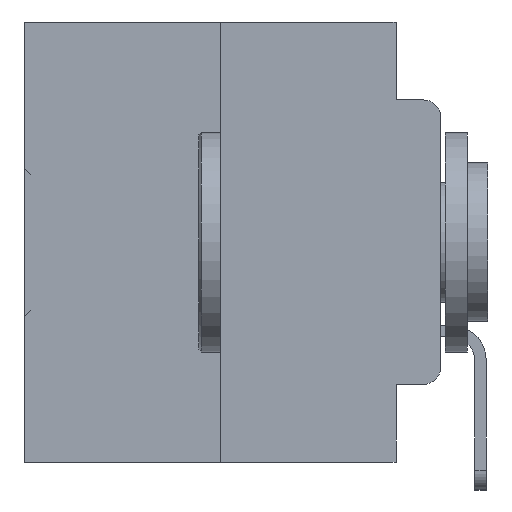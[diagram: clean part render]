
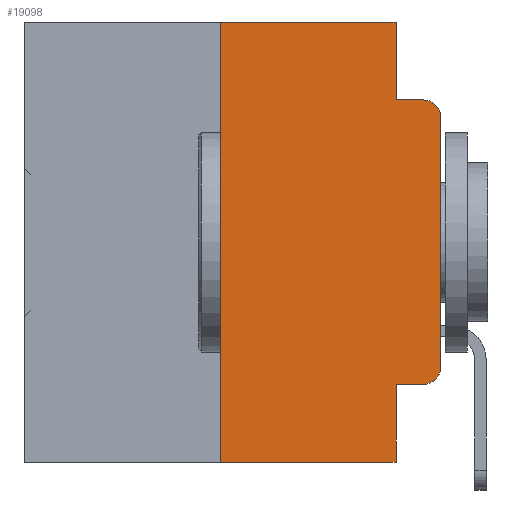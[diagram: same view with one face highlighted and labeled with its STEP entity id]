
A CAD part, left-side view. The second image highlights one B-rep face of the part: STEP entity #19098.
In plain terms, the highlighted planar face has unit normal (-1, 0, 0).
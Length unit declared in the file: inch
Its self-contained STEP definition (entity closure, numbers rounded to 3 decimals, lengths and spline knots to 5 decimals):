
#372 = AXIS2_PLACEMENT_3D ( 'NONE', #493, #19734, #3300 ) ;
#493 = CARTESIAN_POINT ( 'NONE',  ( 0., 0.02, -0.1085 ) ) ;
#809 = DIRECTION ( 'NONE',  ( 0., -1., 0. ) ) ;
#1247 = CARTESIAN_POINT ( 'NONE',  ( 0., 0.25, 0. ) ) ;
#1377 = DIRECTION ( 'NONE',  ( 0., 0., -1. ) ) ;
#1588 = DIRECTION ( 'NONE',  ( 0., 0., -1. ) ) ;
#1633 = CARTESIAN_POINT ( 'NONE',  ( 0., 0.051, -0.0885 ) ) ;
#1712 = CARTESIAN_POINT ( 'NONE',  ( 0., 0.051, 0. ) ) ;
#2643 = AXIS2_PLACEMENT_3D ( 'NONE', #33662, #17865, #1377 ) ;
#2871 = VERTEX_POINT ( 'NONE', #22333 ) ;
#2929 = DIRECTION ( 'NONE',  ( 0., 0., -1. ) ) ;
#3300 = DIRECTION ( 'NONE',  ( 0., 0., -1. ) ) ;
#3422 = EDGE_LOOP ( 'NONE', ( #8498, #23719, #23021, #17663, #18103, #30913, #30508, #13424, #20625, #8719 ) ) ;
#4654 = CARTESIAN_POINT ( 'NONE',  ( 0., 0.02, -0.4115 ) ) ;
#4959 = CARTESIAN_POINT ( 'NONE',  ( 0., 0.051, -0.5 ) ) ;
#5313 = DIRECTION ( 'NONE',  ( 0., -1., 0. ) ) ;
#5554 = DIRECTION ( 'NONE',  ( 0., 0., -1. ) ) ;
#5927 = VERTEX_POINT ( 'NONE', #18514 ) ;
#6428 = CARTESIAN_POINT ( 'NONE',  ( 0., 0.473, -0.5 ) ) ;
#8099 = CARTESIAN_POINT ( 'NONE',  ( 0., 0.473, 0. ) ) ;
#8263 = CARTESIAN_POINT ( 'NONE',  ( 0., 0.473, 0. ) ) ;
#8498 = ORIENTED_EDGE ( 'NONE', *, *, #14385, .T. ) ;
#8561 = VERTEX_POINT ( 'NONE', #28692 ) ;
#8691 = VERTEX_POINT ( 'NONE', #4959 ) ;
#8719 = ORIENTED_EDGE ( 'NONE', *, *, #18761, .T. ) ;
#9183 = VERTEX_POINT ( 'NONE', #18620 ) ;
#10094 = VERTEX_POINT ( 'NONE', #1633 ) ;
#10362 = LINE ( 'NONE', #30928, #16781 ) ;
#10534 = VECTOR ( 'NONE', #1588, 39.37008 ) ;
#10754 = EDGE_CURVE ( 'NONE', #10094, #27818, #10362, .T. ) ;
#11478 = LINE ( 'NONE', #16391, #26593 ) ;
#11793 = LINE ( 'NONE', #14503, #32259 ) ;
#12131 = CARTESIAN_POINT ( 'NONE',  ( 0., 0.25, 0. ) ) ;
#12580 = EDGE_CURVE ( 'NONE', #5927, #27818, #28372, .T. ) ;
#13424 = ORIENTED_EDGE ( 'NONE', *, *, #27581, .F. ) ;
#14385 = EDGE_CURVE ( 'NONE', #8561, #5927, #11478, .T. ) ;
#14503 = CARTESIAN_POINT ( 'NONE',  ( 0., 0.051, -0.4115 ) ) ;
#14835 = AXIS2_PLACEMENT_3D ( 'NONE', #8263, #19368, #2929 ) ;
#15530 = EDGE_CURVE ( 'NONE', #23716, #8691, #27016, .T. ) ;
#16251 = CIRCLE ( 'NONE', #2643, 0.02 ) ;
#16391 = CARTESIAN_POINT ( 'NONE',  ( 0., 0., 0. ) ) ;
#16655 = PLANE ( 'NONE',  #14835 ) ;
#16781 = VECTOR ( 'NONE', #17764, 39.37008 ) ;
#16973 = VECTOR ( 'NONE', #5554, 39.37008 ) ;
#17362 = VECTOR ( 'NONE', #5313, 39.37008 ) ;
#17663 = ORIENTED_EDGE ( 'NONE', *, *, #34643, .F. ) ;
#17764 = DIRECTION ( 'NONE',  ( 0., -1., 0. ) ) ;
#17814 = LINE ( 'NONE', #1712, #10534 ) ;
#17865 = DIRECTION ( 'NONE',  ( -1., 0., 0. ) ) ;
#18103 = ORIENTED_EDGE ( 'NONE', *, *, #34859, .F. ) ;
#18493 = LINE ( 'NONE', #1247, #30865 ) ;
#18514 = CARTESIAN_POINT ( 'NONE',  ( 0., 0., -0.1085 ) ) ;
#18620 = CARTESIAN_POINT ( 'NONE',  ( 0., 0.051, -0.4115 ) ) ;
#18761 = EDGE_CURVE ( 'NONE', #20790, #8561, #16251, .T. ) ;
#19098 = ADVANCED_FACE ( 'NONE', ( #24135 ), #16655, .F. ) ;
#19368 = DIRECTION ( 'NONE',  ( 1., 0., 0. ) ) ;
#19734 = DIRECTION ( 'NONE',  ( -1., 0., 0. ) ) ;
#19964 = DIRECTION ( 'NONE',  ( 0., -1., 0. ) ) ;
#20534 = EDGE_CURVE ( 'NONE', #9183, #20790, #11793, .T. ) ;
#20625 = ORIENTED_EDGE ( 'NONE', *, *, #20534, .T. ) ;
#20790 = VERTEX_POINT ( 'NONE', #4654 ) ;
#22333 = CARTESIAN_POINT ( 'NONE',  ( 0., 0.051, 0. ) ) ;
#23021 = ORIENTED_EDGE ( 'NONE', *, *, #10754, .F. ) ;
#23048 = CARTESIAN_POINT ( 'NONE',  ( 0., 0.25, -0.5 ) ) ;
#23716 = VERTEX_POINT ( 'NONE', #23048 ) ;
#23719 = ORIENTED_EDGE ( 'NONE', *, *, #12580, .T. ) ;
#24135 = FACE_OUTER_BOUND ( 'NONE', #3422, .T. ) ;
#24674 = VECTOR ( 'NONE', #809, 39.37008 ) ;
#25723 = DIRECTION ( 'NONE',  ( 0., 0., 1. ) ) ;
#26593 = VECTOR ( 'NONE', #27050, 39.37008 ) ;
#27016 = LINE ( 'NONE', #6428, #24674 ) ;
#27050 = DIRECTION ( 'NONE',  ( 0., 0., 1. ) ) ;
#27581 = EDGE_CURVE ( 'NONE', #9183, #8691, #31055, .T. ) ;
#27818 = VERTEX_POINT ( 'NONE', #30816 ) ;
#28372 = CIRCLE ( 'NONE', #372, 0.02 ) ;
#28692 = CARTESIAN_POINT ( 'NONE',  ( 0., 0., -0.3915 ) ) ;
#28834 = VERTEX_POINT ( 'NONE', #12131 ) ;
#29349 = EDGE_CURVE ( 'NONE', #23716, #28834, #18493, .T. ) ;
#30508 = ORIENTED_EDGE ( 'NONE', *, *, #15530, .T. ) ;
#30816 = CARTESIAN_POINT ( 'NONE',  ( 0., 0.02, -0.0885 ) ) ;
#30865 = VECTOR ( 'NONE', #25723, 39.37008 ) ;
#30913 = ORIENTED_EDGE ( 'NONE', *, *, #29349, .F. ) ;
#30928 = CARTESIAN_POINT ( 'NONE',  ( 0., 0.051, -0.0885 ) ) ;
#31055 = LINE ( 'NONE', #34977, #16973 ) ;
#31439 = LINE ( 'NONE', #8099, #17362 ) ;
#32259 = VECTOR ( 'NONE', #19964, 39.37008 ) ;
#33662 = CARTESIAN_POINT ( 'NONE',  ( 0., 0.02, -0.3915 ) ) ;
#34643 = EDGE_CURVE ( 'NONE', #2871, #10094, #17814, .T. ) ;
#34859 = EDGE_CURVE ( 'NONE', #28834, #2871, #31439, .T. ) ;
#34977 = CARTESIAN_POINT ( 'NONE',  ( 0., 0.051, 0. ) ) ;
